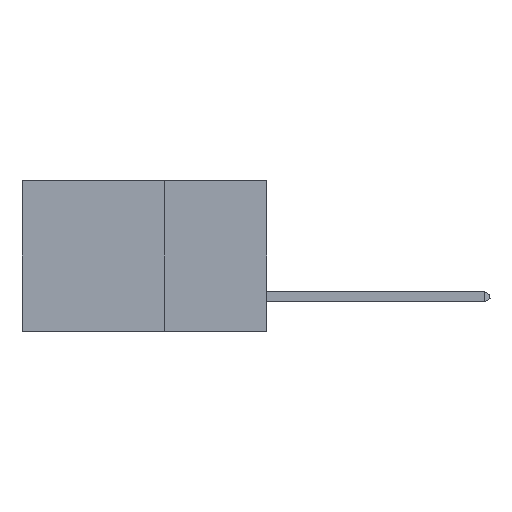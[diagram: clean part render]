
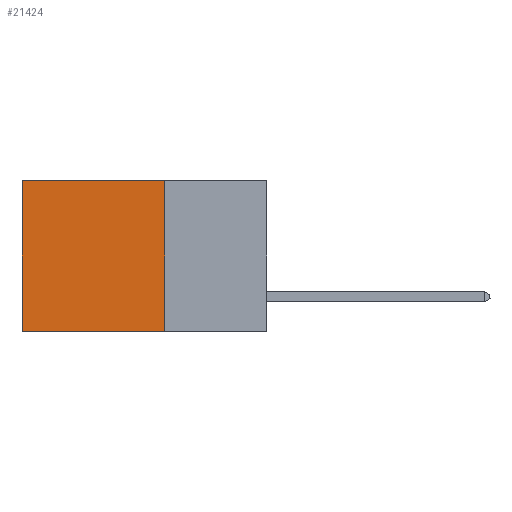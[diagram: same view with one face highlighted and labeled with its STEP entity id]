
A CAD part, left-side view. The second image highlights one B-rep face of the part: STEP entity #21424.
In plain terms, the highlighted planar face has unit normal (-1, 0, 0).
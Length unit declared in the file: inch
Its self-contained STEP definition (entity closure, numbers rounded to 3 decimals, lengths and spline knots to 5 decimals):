
#174 = VERTEX_POINT ( 'NONE', #32013 ) ;
#1086 = DIRECTION ( 'NONE',  ( 0., 0., -1. ) ) ;
#1102 = VECTOR ( 'NONE', #1086, 39.37008 ) ;
#2556 = CARTESIAN_POINT ( 'NONE',  ( 0.2875, 0.6, -0.37 ) ) ;
#4993 = CARTESIAN_POINT ( 'NONE',  ( 0.2875, 0.25, 0. ) ) ;
#6493 = DIRECTION ( 'NONE',  ( 0., 1., 0. ) ) ;
#10090 = VERTEX_POINT ( 'NONE', #31715 ) ;
#10918 = VERTEX_POINT ( 'NONE', #4993 ) ;
#11845 = LINE ( 'NONE', #21494, #1102 ) ;
#12220 = VECTOR ( 'NONE', #29041, 39.37008 ) ;
#13035 = CARTESIAN_POINT ( 'NONE',  ( 0.2875, 0.25, -0.37 ) ) ;
#13568 = ORIENTED_EDGE ( 'NONE', *, *, #43365, .F. ) ;
#15501 = CARTESIAN_POINT ( 'NONE',  ( 0.2875, 0.25, 0. ) ) ;
#15972 = CARTESIAN_POINT ( 'NONE',  ( 0.2875, 0.6, 0. ) ) ;
#16237 = LINE ( 'NONE', #26826, #43367 ) ;
#17317 = EDGE_CURVE ( 'NONE', #10090, #35905, #18518, .T. ) ;
#17373 = ORIENTED_EDGE ( 'NONE', *, *, #22985, .F. ) ;
#18518 = LINE ( 'NONE', #15972, #12220 ) ;
#18895 = DIRECTION ( 'NONE',  ( 0., 0., -1. ) ) ;
#19595 = FACE_OUTER_BOUND ( 'NONE', #37531, .T. ) ;
#21424 = ADVANCED_FACE ( 'NONE', ( #19595 ), #35902, .F. ) ;
#21494 = CARTESIAN_POINT ( 'NONE',  ( 0.2875, 0.25, 0. ) ) ;
#22985 = EDGE_CURVE ( 'NONE', #174, #35905, #39760, .T. ) ;
#23590 = ORIENTED_EDGE ( 'NONE', *, *, #17317, .T. ) ;
#26826 = CARTESIAN_POINT ( 'NONE',  ( 0.2875, 0.25, 0. ) ) ;
#26887 = AXIS2_PLACEMENT_3D ( 'NONE', #15501, #39290, #18895 ) ;
#27232 = DIRECTION ( 'NONE',  ( 0., 1., 0. ) ) ;
#29041 = DIRECTION ( 'NONE',  ( 0., 0., -1. ) ) ;
#31715 = CARTESIAN_POINT ( 'NONE',  ( 0.2875, 0.6, 0. ) ) ;
#32013 = CARTESIAN_POINT ( 'NONE',  ( 0.2875, 0.25, -0.37 ) ) ;
#34433 = VECTOR ( 'NONE', #27232, 39.37008 ) ;
#35902 = PLANE ( 'NONE',  #26887 ) ;
#35905 = VERTEX_POINT ( 'NONE', #2556 ) ;
#36796 = ORIENTED_EDGE ( 'NONE', *, *, #36801, .T. ) ;
#36801 = EDGE_CURVE ( 'NONE', #10918, #10090, #16237, .T. ) ;
#37531 = EDGE_LOOP ( 'NONE', ( #23590, #17373, #13568, #36796 ) ) ;
#39290 = DIRECTION ( 'NONE',  ( 1., 0., 0. ) ) ;
#39760 = LINE ( 'NONE', #13035, #34433 ) ;
#43365 = EDGE_CURVE ( 'NONE', #10918, #174, #11845, .T. ) ;
#43367 = VECTOR ( 'NONE', #6493, 39.37008 ) ;
